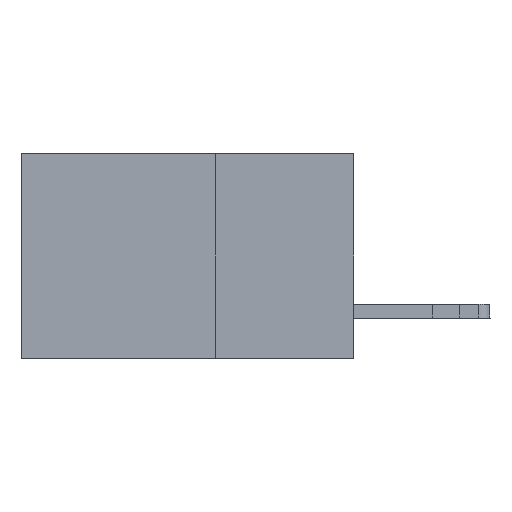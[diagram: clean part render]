
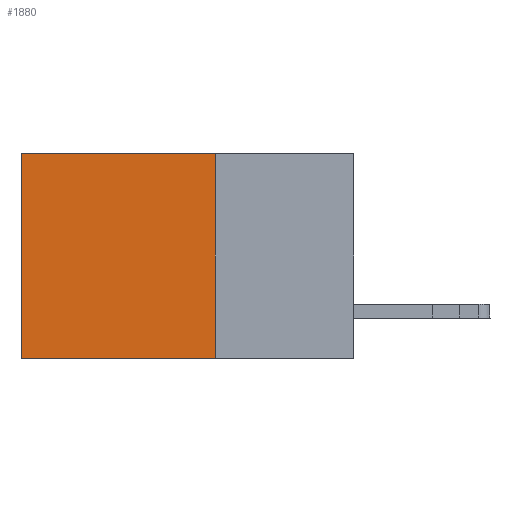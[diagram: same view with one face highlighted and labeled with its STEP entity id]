
A CAD part, left-side view. The second image highlights one B-rep face of the part: STEP entity #1880.
In plain terms, the highlighted planar face has unit normal (-1, 0, 0).
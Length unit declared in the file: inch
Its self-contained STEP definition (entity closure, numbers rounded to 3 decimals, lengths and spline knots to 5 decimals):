
#978 = EDGE_CURVE ( 'NONE', #16683, #15286, #19445, .T. ) ;
#1192 = DIRECTION ( 'NONE',  ( 0., 0., -1. ) ) ;
#1653 = CARTESIAN_POINT ( 'NONE',  ( 0.2875, 0.6, -0.37 ) ) ;
#1880 = ADVANCED_FACE ( 'NONE', ( #3564 ), #11574, .F. ) ;
#1915 = DIRECTION ( 'NONE',  ( 0., 1., 0. ) ) ;
#2185 = EDGE_CURVE ( 'NONE', #10526, #16751, #15208, .T. ) ;
#2654 = CARTESIAN_POINT ( 'NONE',  ( 0.2875, 0.25, -0.37 ) ) ;
#3564 = FACE_OUTER_BOUND ( 'NONE', #19821, .T. ) ;
#6325 = AXIS2_PLACEMENT_3D ( 'NONE', #17654, #13635, #1192 ) ;
#7563 = CARTESIAN_POINT ( 'NONE',  ( 0.2875, 0.25, -0.37 ) ) ;
#7690 = ORIENTED_EDGE ( 'NONE', *, *, #978, .F. ) ;
#8910 = VECTOR ( 'NONE', #13826, 39.37008 ) ;
#9751 = VECTOR ( 'NONE', #17020, 39.37008 ) ;
#10526 = VERTEX_POINT ( 'NONE', #13668 ) ;
#11574 = PLANE ( 'NONE',  #6325 ) ;
#12574 = ORIENTED_EDGE ( 'NONE', *, *, #18552, .F. ) ;
#12619 = EDGE_CURVE ( 'NONE', #16683, #10526, #18994, .T. ) ;
#12908 = CARTESIAN_POINT ( 'NONE',  ( 0.2875, 0.6, 0. ) ) ;
#13372 = VECTOR ( 'NONE', #20935, 39.37008 ) ;
#13489 = ORIENTED_EDGE ( 'NONE', *, *, #12619, .T. ) ;
#13563 = VECTOR ( 'NONE', #1915, 39.37008 ) ;
#13635 = DIRECTION ( 'NONE',  ( 1., 0., 0. ) ) ;
#13668 = CARTESIAN_POINT ( 'NONE',  ( 0.2875, 0.6, 0. ) ) ;
#13826 = DIRECTION ( 'NONE',  ( 0., 1., 0. ) ) ;
#14370 = LINE ( 'NONE', #7563, #8910 ) ;
#15208 = LINE ( 'NONE', #12908, #9751 ) ;
#15286 = VERTEX_POINT ( 'NONE', #2654 ) ;
#15922 = ORIENTED_EDGE ( 'NONE', *, *, #2185, .T. ) ;
#16683 = VERTEX_POINT ( 'NONE', #21979 ) ;
#16751 = VERTEX_POINT ( 'NONE', #1653 ) ;
#17020 = DIRECTION ( 'NONE',  ( 0., 0., -1. ) ) ;
#17654 = CARTESIAN_POINT ( 'NONE',  ( 0.2875, 0.25, 0. ) ) ;
#18552 = EDGE_CURVE ( 'NONE', #15286, #16751, #14370, .T. ) ;
#18994 = LINE ( 'NONE', #20432, #13563 ) ;
#19445 = LINE ( 'NONE', #21108, #13372 ) ;
#19821 = EDGE_LOOP ( 'NONE', ( #15922, #12574, #7690, #13489 ) ) ;
#20432 = CARTESIAN_POINT ( 'NONE',  ( 0.2875, 0.25, 0. ) ) ;
#20935 = DIRECTION ( 'NONE',  ( 0., 0., -1. ) ) ;
#21108 = CARTESIAN_POINT ( 'NONE',  ( 0.2875, 0.25, 0. ) ) ;
#21979 = CARTESIAN_POINT ( 'NONE',  ( 0.2875, 0.25, 0. ) ) ;
